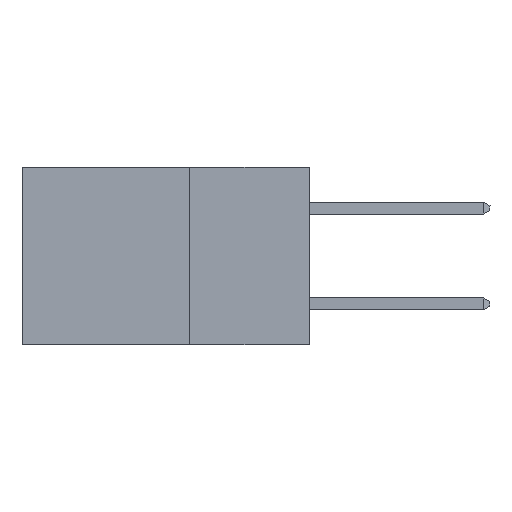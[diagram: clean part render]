
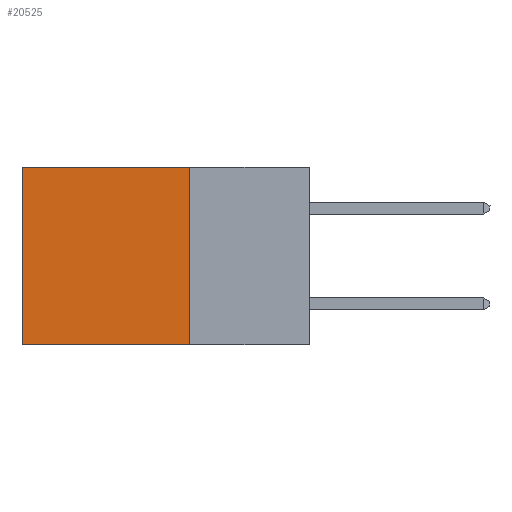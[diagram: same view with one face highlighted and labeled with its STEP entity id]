
A CAD part, left-side view. The second image highlights one B-rep face of the part: STEP entity #20525.
In plain terms, the highlighted planar face has unit normal (-1, 0, 0).
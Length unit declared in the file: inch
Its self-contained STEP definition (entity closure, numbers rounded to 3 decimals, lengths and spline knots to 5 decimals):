
#514 = DIRECTION ( 'NONE',  ( 0., 1., 0. ) ) ;
#530 = LINE ( 'NONE', #13434, #23643 ) ;
#1635 = CARTESIAN_POINT ( 'NONE',  ( 0.2875, 0.25, -0.37 ) ) ;
#2671 = CARTESIAN_POINT ( 'NONE',  ( 0.2875, 0.25, 0. ) ) ;
#3757 = EDGE_LOOP ( 'NONE', ( #14695, #8722, #20812, #11925 ) ) ;
#4508 = DIRECTION ( 'NONE',  ( 1., 0., 0. ) ) ;
#5363 = VERTEX_POINT ( 'NONE', #11451 ) ;
#5630 = LINE ( 'NONE', #14501, #19542 ) ;
#6476 = CARTESIAN_POINT ( 'NONE',  ( 0.2875, 0.6, -0.37 ) ) ;
#7558 = CARTESIAN_POINT ( 'NONE',  ( 0.2875, 0.6, 0. ) ) ;
#7814 = EDGE_CURVE ( 'NONE', #13454, #16797, #19860, .T. ) ;
#8121 = PLANE ( 'NONE',  #17549 ) ;
#8722 = ORIENTED_EDGE ( 'NONE', *, *, #14330, .F. ) ;
#9728 = VERTEX_POINT ( 'NONE', #1635 ) ;
#11451 = CARTESIAN_POINT ( 'NONE',  ( 0.2875, 0.25, 0. ) ) ;
#11823 = DIRECTION ( 'NONE',  ( 0., 1., 0. ) ) ;
#11925 = ORIENTED_EDGE ( 'NONE', *, *, #19583, .T. ) ;
#12658 = FACE_OUTER_BOUND ( 'NONE', #3757, .T. ) ;
#13434 = CARTESIAN_POINT ( 'NONE',  ( 0.2875, 0.25, 0. ) ) ;
#13454 = VERTEX_POINT ( 'NONE', #17518 ) ;
#14330 = EDGE_CURVE ( 'NONE', #9728, #16797, #21301, .T. ) ;
#14501 = CARTESIAN_POINT ( 'NONE',  ( 0.2875, 0.25, 0. ) ) ;
#14695 = ORIENTED_EDGE ( 'NONE', *, *, #7814, .T. ) ;
#16313 = DIRECTION ( 'NONE',  ( 0., 0., -1. ) ) ;
#16565 = VECTOR ( 'NONE', #11823, 39.37008 ) ;
#16797 = VERTEX_POINT ( 'NONE', #6476 ) ;
#17222 = DIRECTION ( 'NONE',  ( 0., 0., -1. ) ) ;
#17518 = CARTESIAN_POINT ( 'NONE',  ( 0.2875, 0.6, 0. ) ) ;
#17549 = AXIS2_PLACEMENT_3D ( 'NONE', #2671, #4508, #17222 ) ;
#19542 = VECTOR ( 'NONE', #16313, 39.37008 ) ;
#19583 = EDGE_CURVE ( 'NONE', #5363, #13454, #530, .T. ) ;
#19860 = LINE ( 'NONE', #7558, #20430 ) ;
#20170 = DIRECTION ( 'NONE',  ( 0., 0., -1. ) ) ;
#20430 = VECTOR ( 'NONE', #20170, 39.37008 ) ;
#20525 = ADVANCED_FACE ( 'NONE', ( #12658 ), #8121, .F. ) ;
#20812 = ORIENTED_EDGE ( 'NONE', *, *, #22066, .F. ) ;
#20822 = CARTESIAN_POINT ( 'NONE',  ( 0.2875, 0.25, -0.37 ) ) ;
#21301 = LINE ( 'NONE', #20822, #16565 ) ;
#22066 = EDGE_CURVE ( 'NONE', #5363, #9728, #5630, .T. ) ;
#23643 = VECTOR ( 'NONE', #514, 39.37008 ) ;
